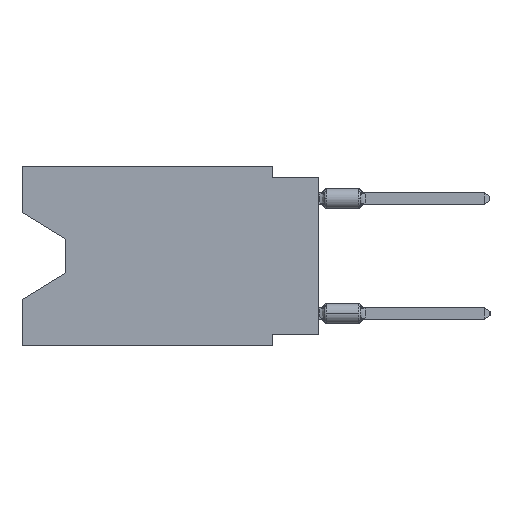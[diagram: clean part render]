
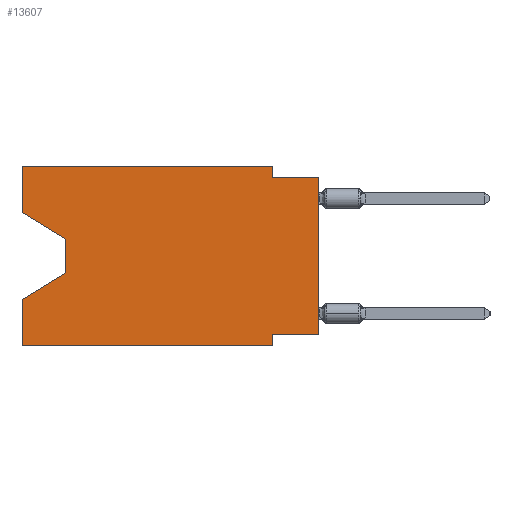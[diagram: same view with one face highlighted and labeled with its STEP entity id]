
A CAD part, left-side view. The second image highlights one B-rep face of the part: STEP entity #13607.
In plain terms, the highlighted planar face has unit normal (-1, 0, 0).
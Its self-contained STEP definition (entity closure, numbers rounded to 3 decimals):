
#410 = VERTEX_POINT ( 'NONE', #44192 ) ;
#993 = LINE ( 'NONE', #19650, #44670 ) ;
#2057 = VERTEX_POINT ( 'NONE', #5917 ) ;
#2186 = LINE ( 'NONE', #12252, #42778 ) ;
#2225 = LINE ( 'NONE', #22200, #25685 ) ;
#2452 = DIRECTION ( 'NONE',  ( 0., 0., -1. ) ) ;
#2528 = CARTESIAN_POINT ( 'NONE',  ( 0., 16.383, -9.906 ) ) ;
#3934 = DIRECTION ( 'NONE',  ( 0., 0., -1. ) ) ;
#4354 = ORIENTED_EDGE ( 'NONE', *, *, #10658, .T. ) ;
#4589 = DIRECTION ( 'NONE',  ( 0., 0., 1. ) ) ;
#4697 = VECTOR ( 'NONE', #37337, 1000. ) ;
#5872 = LINE ( 'NONE', #19817, #38488 ) ;
#5917 = CARTESIAN_POINT ( 'NONE',  ( 0., 2.54, 0. ) ) ;
#5938 = CARTESIAN_POINT ( 'NONE',  ( 0., 16.383, -9.906 ) ) ;
#7565 = VECTOR ( 'NONE', #13103, 1000. ) ;
#8608 = DIRECTION ( 'NONE',  ( 0., 0.855, -0.519 ) ) ;
#8735 = CARTESIAN_POINT ( 'NONE',  ( 0., 16.383, -7.36 ) ) ;
#9373 = DIRECTION ( 'NONE',  ( 0., 0., 1. ) ) ;
#10121 = ORIENTED_EDGE ( 'NONE', *, *, #36539, .F. ) ;
#10396 = LINE ( 'NONE', #34657, #43247 ) ;
#10607 = ORIENTED_EDGE ( 'NONE', *, *, #11511, .F. ) ;
#10658 = EDGE_CURVE ( 'NONE', #21847, #410, #37284, .T. ) ;
#11154 = PLANE ( 'NONE',  #12028 ) ;
#11511 = EDGE_CURVE ( 'NONE', #12554, #17789, #23182, .T. ) ;
#11991 = CARTESIAN_POINT ( 'NONE',  ( 0., 2.54, -9.271 ) ) ;
#12028 = AXIS2_PLACEMENT_3D ( 'NONE', #13892, #38843, #35409 ) ;
#12252 = CARTESIAN_POINT ( 'NONE',  ( 0., 13.97, -5.893 ) ) ;
#12554 = VERTEX_POINT ( 'NONE', #25779 ) ;
#13072 = EDGE_LOOP ( 'NONE', ( #15483, #39266, #37584, #26011, #4354, #19253, #13422, #22547, #10607, #40410, #23467, #10121 ) ) ;
#13103 = DIRECTION ( 'NONE',  ( 0., -1., 0. ) ) ;
#13350 = DIRECTION ( 'NONE',  ( 0., -1., 0. ) ) ;
#13422 = ORIENTED_EDGE ( 'NONE', *, *, #25735, .F. ) ;
#13451 = VECTOR ( 'NONE', #3934, 1000. ) ;
#13607 = ADVANCED_FACE ( 'NONE', ( #31289 ), #11154, .F. ) ;
#13892 = CARTESIAN_POINT ( 'NONE',  ( 0., 16.383, 0. ) ) ;
#14017 = LINE ( 'NONE', #20657, #37606 ) ;
#14384 = CARTESIAN_POINT ( 'NONE',  ( 0., 13.97, -4.013 ) ) ;
#14883 = EDGE_CURVE ( 'NONE', #21847, #39911, #2225, .T. ) ;
#15483 = ORIENTED_EDGE ( 'NONE', *, *, #28162, .T. ) ;
#15536 = DIRECTION ( 'NONE',  ( 0., 0., 1. ) ) ;
#16334 = VERTEX_POINT ( 'NONE', #41397 ) ;
#17789 = VERTEX_POINT ( 'NONE', #25595 ) ;
#19253 = ORIENTED_EDGE ( 'NONE', *, *, #41739, .F. ) ;
#19650 = CARTESIAN_POINT ( 'NONE',  ( 0., 16.383, 0. ) ) ;
#19817 = CARTESIAN_POINT ( 'NONE',  ( 0., 13.97, -4.013 ) ) ;
#19893 = DIRECTION ( 'NONE',  ( 0., -1., 0. ) ) ;
#20081 = DIRECTION ( 'NONE',  ( 0., 0., -1. ) ) ;
#20657 = CARTESIAN_POINT ( 'NONE',  ( 0., 16.383, 0. ) ) ;
#21710 = EDGE_CURVE ( 'NONE', #2057, #12554, #22444, .T. ) ;
#21847 = VERTEX_POINT ( 'NONE', #2528 ) ;
#22200 = CARTESIAN_POINT ( 'NONE',  ( 0., 16.383, 0. ) ) ;
#22444 = LINE ( 'NONE', #39173, #13451 ) ;
#22547 = ORIENTED_EDGE ( 'NONE', *, *, #40299, .T. ) ;
#23086 = LINE ( 'NONE', #37040, #27974 ) ;
#23182 = LINE ( 'NONE', #23861, #7565 ) ;
#23467 = ORIENTED_EDGE ( 'NONE', *, *, #30446, .F. ) ;
#23861 = CARTESIAN_POINT ( 'NONE',  ( 0., 0., -0.635 ) ) ;
#24138 = DIRECTION ( 'NONE',  ( 0., 1., 0. ) ) ;
#25595 = CARTESIAN_POINT ( 'NONE',  ( 0., 0., -0.635 ) ) ;
#25685 = VECTOR ( 'NONE', #4589, 1000. ) ;
#25735 = EDGE_CURVE ( 'NONE', #35919, #42411, #10396, .T. ) ;
#25779 = CARTESIAN_POINT ( 'NONE',  ( 0., 2.54, -0.635 ) ) ;
#26011 = ORIENTED_EDGE ( 'NONE', *, *, #14883, .F. ) ;
#26447 = VERTEX_POINT ( 'NONE', #33294 ) ;
#26832 = VECTOR ( 'NONE', #20081, 1000. ) ;
#27042 = CARTESIAN_POINT ( 'NONE',  ( 0., 16.383, -2.546 ) ) ;
#27238 = VECTOR ( 'NONE', #19893, 1000. ) ;
#27974 = VECTOR ( 'NONE', #15536, 1000. ) ;
#28162 = EDGE_CURVE ( 'NONE', #16334, #28750, #36900, .T. ) ;
#28750 = VERTEX_POINT ( 'NONE', #14384 ) ;
#29270 = EDGE_CURVE ( 'NONE', #30448, #39911, #2186, .T. ) ;
#30446 = EDGE_CURVE ( 'NONE', #26447, #2057, #14017, .T. ) ;
#30448 = VERTEX_POINT ( 'NONE', #44924 ) ;
#30825 = CARTESIAN_POINT ( 'NONE',  ( 0., 2.54, -9.906 ) ) ;
#31289 = FACE_OUTER_BOUND ( 'NONE', #13072, .T. ) ;
#32891 = EDGE_CURVE ( 'NONE', #28750, #30448, #5872, .T. ) ;
#33294 = CARTESIAN_POINT ( 'NONE',  ( 0., 16.383, 0. ) ) ;
#34657 = CARTESIAN_POINT ( 'NONE',  ( 0., 0., -9.271 ) ) ;
#35409 = DIRECTION ( 'NONE',  ( 0., 0., -1. ) ) ;
#35919 = VERTEX_POINT ( 'NONE', #44535 ) ;
#36539 = EDGE_CURVE ( 'NONE', #16334, #26447, #993, .T. ) ;
#36900 = LINE ( 'NONE', #27042, #4697 ) ;
#37040 = CARTESIAN_POINT ( 'NONE',  ( 0., 0., 0. ) ) ;
#37284 = LINE ( 'NONE', #5938, #27238 ) ;
#37337 = DIRECTION ( 'NONE',  ( 0., -0.855, -0.519 ) ) ;
#37584 = ORIENTED_EDGE ( 'NONE', *, *, #29270, .T. ) ;
#37606 = VECTOR ( 'NONE', #13350, 1000. ) ;
#37695 = LINE ( 'NONE', #30825, #26832 ) ;
#38488 = VECTOR ( 'NONE', #2452, 1000. ) ;
#38843 = DIRECTION ( 'NONE',  ( 1., 0., 0. ) ) ;
#39173 = CARTESIAN_POINT ( 'NONE',  ( 0., 2.54, 0. ) ) ;
#39266 = ORIENTED_EDGE ( 'NONE', *, *, #32891, .T. ) ;
#39911 = VERTEX_POINT ( 'NONE', #8735 ) ;
#40299 = EDGE_CURVE ( 'NONE', #35919, #17789, #23086, .T. ) ;
#40410 = ORIENTED_EDGE ( 'NONE', *, *, #21710, .F. ) ;
#41397 = CARTESIAN_POINT ( 'NONE',  ( 0., 16.383, -2.546 ) ) ;
#41739 = EDGE_CURVE ( 'NONE', #42411, #410, #37695, .T. ) ;
#42411 = VERTEX_POINT ( 'NONE', #11991 ) ;
#42778 = VECTOR ( 'NONE', #8608, 1000. ) ;
#43247 = VECTOR ( 'NONE', #24138, 1000. ) ;
#44192 = CARTESIAN_POINT ( 'NONE',  ( 0., 2.54, -9.906 ) ) ;
#44535 = CARTESIAN_POINT ( 'NONE',  ( 0., 0., -9.271 ) ) ;
#44670 = VECTOR ( 'NONE', #9373, 1000. ) ;
#44924 = CARTESIAN_POINT ( 'NONE',  ( 0., 13.97, -5.893 ) ) ;
